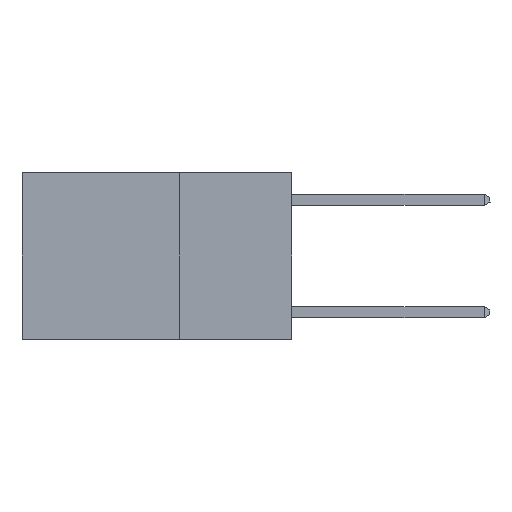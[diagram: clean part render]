
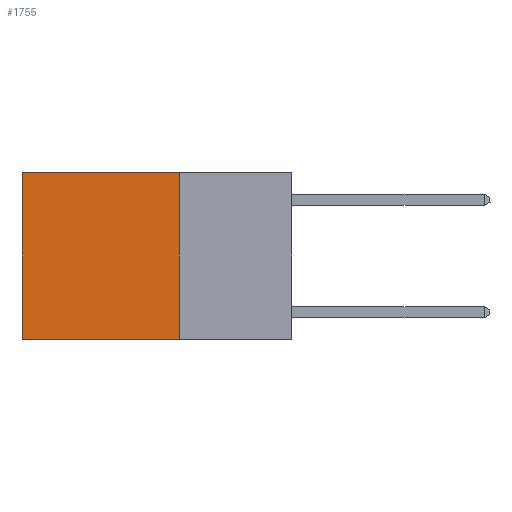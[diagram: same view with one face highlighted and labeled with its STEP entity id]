
A CAD part, left-side view. The second image highlights one B-rep face of the part: STEP entity #1755.
In plain terms, the highlighted planar face has unit normal (-1, 0, 0).
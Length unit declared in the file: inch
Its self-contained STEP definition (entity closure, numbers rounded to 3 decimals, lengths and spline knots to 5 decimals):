
#69 = VECTOR ( 'NONE', #19527, 39.37008 ) ;
#626 = CARTESIAN_POINT ( 'NONE',  ( 0.2625, 0.25, 0. ) ) ;
#668 = VERTEX_POINT ( 'NONE', #1227 ) ;
#974 = CARTESIAN_POINT ( 'NONE',  ( 0.2625, 0.6, 0. ) ) ;
#1227 = CARTESIAN_POINT ( 'NONE',  ( 0.2625, 0.25, 0. ) ) ;
#1755 = ADVANCED_FACE ( 'NONE', ( #14915 ), #3515, .F. ) ;
#1803 = VERTEX_POINT ( 'NONE', #19059 ) ;
#2313 = EDGE_CURVE ( 'NONE', #17375, #1803, #6086, .T. ) ;
#2928 = LINE ( 'NONE', #7297, #69 ) ;
#3515 = PLANE ( 'NONE',  #12716 ) ;
#3646 = DIRECTION ( 'NONE',  ( 0., 0., -1. ) ) ;
#4677 = CARTESIAN_POINT ( 'NONE',  ( 0.2625, 0.25, -0.37 ) ) ;
#5373 = CARTESIAN_POINT ( 'NONE',  ( 0.2625, 0.25, -0.37 ) ) ;
#5657 = ORIENTED_EDGE ( 'NONE', *, *, #8457, .T. ) ;
#5706 = VECTOR ( 'NONE', #8556, 39.37008 ) ;
#5802 = CARTESIAN_POINT ( 'NONE',  ( 0.2625, 0.6, 0. ) ) ;
#6086 = LINE ( 'NONE', #4677, #17806 ) ;
#6203 = LINE ( 'NONE', #974, #5706 ) ;
#6275 = DIRECTION ( 'NONE',  ( 0., 1., 0. ) ) ;
#7297 = CARTESIAN_POINT ( 'NONE',  ( 0.2625, 0.25, 0. ) ) ;
#8457 = EDGE_CURVE ( 'NONE', #668, #19275, #16126, .T. ) ;
#8556 = DIRECTION ( 'NONE',  ( 0., 0., -1. ) ) ;
#8595 = EDGE_CURVE ( 'NONE', #19275, #1803, #6203, .T. ) ;
#8702 = VECTOR ( 'NONE', #6275, 39.37008 ) ;
#12318 = ORIENTED_EDGE ( 'NONE', *, *, #19380, .F. ) ;
#12716 = AXIS2_PLACEMENT_3D ( 'NONE', #626, #14195, #3646 ) ;
#12798 = ORIENTED_EDGE ( 'NONE', *, *, #2313, .F. ) ;
#13290 = ORIENTED_EDGE ( 'NONE', *, *, #8595, .T. ) ;
#14195 = DIRECTION ( 'NONE',  ( 1., 0., 0. ) ) ;
#14915 = FACE_OUTER_BOUND ( 'NONE', #17529, .T. ) ;
#16126 = LINE ( 'NONE', #18364, #8702 ) ;
#17375 = VERTEX_POINT ( 'NONE', #5373 ) ;
#17529 = EDGE_LOOP ( 'NONE', ( #13290, #12798, #12318, #5657 ) ) ;
#17806 = VECTOR ( 'NONE', #19671, 39.37008 ) ;
#18364 = CARTESIAN_POINT ( 'NONE',  ( 0.2625, 0.25, 0. ) ) ;
#19059 = CARTESIAN_POINT ( 'NONE',  ( 0.2625, 0.6, -0.37 ) ) ;
#19275 = VERTEX_POINT ( 'NONE', #5802 ) ;
#19380 = EDGE_CURVE ( 'NONE', #668, #17375, #2928, .T. ) ;
#19527 = DIRECTION ( 'NONE',  ( 0., 0., -1. ) ) ;
#19671 = DIRECTION ( 'NONE',  ( 0., 1., 0. ) ) ;
